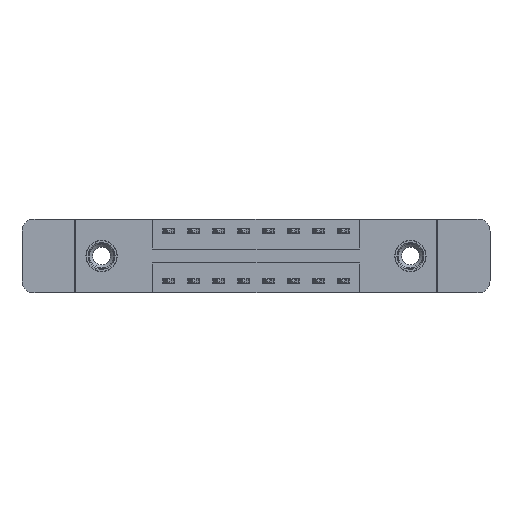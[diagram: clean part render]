
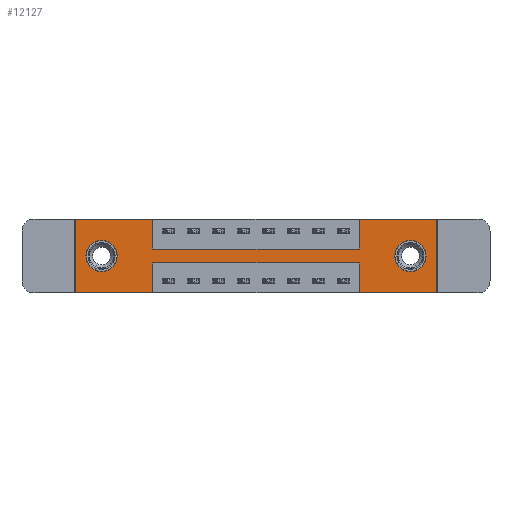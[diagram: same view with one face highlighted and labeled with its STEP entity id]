
A CAD part, front view. The second image highlights one B-rep face of the part: STEP entity #12127.
In plain terms, the highlighted planar face has unit normal (0, -1, 0).
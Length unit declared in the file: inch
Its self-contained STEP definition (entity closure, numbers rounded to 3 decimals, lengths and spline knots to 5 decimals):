
#292 = DIRECTION ( 'NONE',  ( 1., 0., 0. ) ) ;
#681 = CARTESIAN_POINT ( 'NONE',  ( 1.4225, 0., -0.37 ) ) ;
#776 = VERTEX_POINT ( 'NONE', #7445 ) ;
#814 = ORIENTED_EDGE ( 'NONE', *, *, #9265, .T. ) ;
#912 = VECTOR ( 'NONE', #6201, 39.37008 ) ;
#987 = DIRECTION ( 'NONE',  ( 0., 0., -1. ) ) ;
#1143 = PLANE ( 'NONE',  #5718 ) ;
#1169 = CARTESIAN_POINT ( 'NONE',  ( 0., 0., 0. ) ) ;
#1206 = DIRECTION ( 'NONE',  ( -1., 0., 0. ) ) ;
#1479 = EDGE_CURVE ( 'NONE', #11571, #13150, #12919, .T. ) ;
#1709 = ORIENTED_EDGE ( 'NONE', *, *, #5770, .F. ) ;
#1816 = DIRECTION ( 'NONE',  ( 0., 1., 0. ) ) ;
#1830 = ORIENTED_EDGE ( 'NONE', *, *, #4069, .F. ) ;
#1950 = VERTEX_POINT ( 'NONE', #3551 ) ;
#2066 = EDGE_CURVE ( 'NONE', #13150, #11571, #7248, .T. ) ;
#2183 = DIRECTION ( 'NONE',  ( 0., 0., -1. ) ) ;
#2210 = ORIENTED_EDGE ( 'NONE', *, *, #11761, .F. ) ;
#2298 = AXIS2_PLACEMENT_3D ( 'NONE', #3751, #12942, #4683 ) ;
#2528 = CARTESIAN_POINT ( 'NONE',  ( 0., 0., -0.37 ) ) ;
#2551 = DIRECTION ( 'NONE',  ( 0., -1., 0. ) ) ;
#3157 = EDGE_CURVE ( 'NONE', #13590, #13676, #3635, .T. ) ;
#3360 = CARTESIAN_POINT ( 'NONE',  ( 0.1325, 0., -0.107 ) ) ;
#3379 = VERTEX_POINT ( 'NONE', #6526 ) ;
#3422 = CIRCLE ( 'NONE', #5685, 0.078 ) ;
#3471 = VECTOR ( 'NONE', #6344, 39.37008 ) ;
#3551 = CARTESIAN_POINT ( 'NONE',  ( 0.3875, 0., -0.37 ) ) ;
#3635 = LINE ( 'NONE', #8270, #8037 ) ;
#3661 = VECTOR ( 'NONE', #12760, 39.37008 ) ;
#3684 = LINE ( 'NONE', #7225, #14088 ) ;
#3749 = AXIS2_PLACEMENT_3D ( 'NONE', #9615, #14564, #7372 ) ;
#3751 = CARTESIAN_POINT ( 'NONE',  ( 0.1325, 0., -0.185 ) ) ;
#4069 = EDGE_CURVE ( 'NONE', #776, #15091, #3684, .T. ) ;
#4244 = DIRECTION ( 'NONE',  ( 0., 0., 1. ) ) ;
#4287 = EDGE_CURVE ( 'NONE', #8488, #13590, #7455, .T. ) ;
#4439 = ORIENTED_EDGE ( 'NONE', *, *, #14115, .F. ) ;
#4582 = CARTESIAN_POINT ( 'NONE',  ( 1.4225, 0., 0. ) ) ;
#4631 = CARTESIAN_POINT ( 'NONE',  ( 1.4225, 0., 0. ) ) ;
#4674 = LINE ( 'NONE', #10520, #13749 ) ;
#4681 = VECTOR ( 'NONE', #292, 39.37008 ) ;
#4683 = DIRECTION ( 'NONE',  ( 0., 0., 1. ) ) ;
#4753 = CARTESIAN_POINT ( 'NONE',  ( 0., 0., -0.37 ) ) ;
#4797 = VERTEX_POINT ( 'NONE', #4631 ) ;
#4828 = ORIENTED_EDGE ( 'NONE', *, *, #12594, .F. ) ;
#4850 = LINE ( 'NONE', #8381, #8922 ) ;
#5213 = VERTEX_POINT ( 'NONE', #3360 ) ;
#5369 = VERTEX_POINT ( 'NONE', #9388 ) ;
#5603 = EDGE_CURVE ( 'NONE', #1950, #11584, #5709, .T. ) ;
#5670 = VERTEX_POINT ( 'NONE', #13775 ) ;
#5685 = AXIS2_PLACEMENT_3D ( 'NONE', #15165, #1816, #4244 ) ;
#5709 = LINE ( 'NONE', #14878, #10651 ) ;
#5718 = AXIS2_PLACEMENT_3D ( 'NONE', #4753, #2551, #10680 ) ;
#5770 = EDGE_CURVE ( 'NONE', #5670, #3379, #4674, .T. ) ;
#5925 = ORIENTED_EDGE ( 'NONE', *, *, #7505, .T. ) ;
#6201 = DIRECTION ( 'NONE',  ( 0., 0., 1. ) ) ;
#6270 = EDGE_CURVE ( 'NONE', #9476, #4797, #15256, .T. ) ;
#6344 = DIRECTION ( 'NONE',  ( 0., 0., 1. ) ) ;
#6373 = DIRECTION ( 'NONE',  ( 0., 1., 0. ) ) ;
#6526 = CARTESIAN_POINT ( 'NONE',  ( 1.81, 0., -0.37 ) ) ;
#6554 = EDGE_LOOP ( 'NONE', ( #11236, #10657 ) ) ;
#7031 = DIRECTION ( 'NONE',  ( 0., 0., 1. ) ) ;
#7146 = LINE ( 'NONE', #1169, #3471 ) ;
#7225 = CARTESIAN_POINT ( 'NONE',  ( 0.3875, 0., 0. ) ) ;
#7248 = CIRCLE ( 'NONE', #14914, 0.078 ) ;
#7279 = ORIENTED_EDGE ( 'NONE', *, *, #14817, .F. ) ;
#7372 = DIRECTION ( 'NONE',  ( 0., 0., -1. ) ) ;
#7409 = CARTESIAN_POINT ( 'NONE',  ( 1.6775, 0., -0.185 ) ) ;
#7445 = CARTESIAN_POINT ( 'NONE',  ( 0.3875, 0., 0. ) ) ;
#7455 = LINE ( 'NONE', #13542, #912 ) ;
#7505 = EDGE_CURVE ( 'NONE', #5213, #5369, #9033, .T. ) ;
#7534 = CARTESIAN_POINT ( 'NONE',  ( 1.4225, 0., -0.15 ) ) ;
#7692 = ORIENTED_EDGE ( 'NONE', *, *, #5603, .F. ) ;
#8037 = VECTOR ( 'NONE', #9661, 39.37008 ) ;
#8116 = LINE ( 'NONE', #12607, #3661 ) ;
#8212 = CARTESIAN_POINT ( 'NONE',  ( 1.6775, 0., -0.263 ) ) ;
#8226 = DIRECTION ( 'NONE',  ( 0., 0., -1. ) ) ;
#8270 = CARTESIAN_POINT ( 'NONE',  ( 0.3875, 0., -0.22 ) ) ;
#8381 = CARTESIAN_POINT ( 'NONE',  ( 0.3875, 0., -0.37 ) ) ;
#8488 = VERTEX_POINT ( 'NONE', #681 ) ;
#8575 = LINE ( 'NONE', #2528, #8892 ) ;
#8584 = VECTOR ( 'NONE', #7031, 39.37008 ) ;
#8851 = DIRECTION ( 'NONE',  ( 0., 0., -1. ) ) ;
#8892 = VECTOR ( 'NONE', #1206, 39.37008 ) ;
#8922 = VECTOR ( 'NONE', #8226, 39.37008 ) ;
#8927 = EDGE_CURVE ( 'NONE', #4797, #5670, #8116, .T. ) ;
#9033 = CIRCLE ( 'NONE', #2298, 0.078 ) ;
#9265 = EDGE_CURVE ( 'NONE', #5369, #5213, #3422, .T. ) ;
#9388 = CARTESIAN_POINT ( 'NONE',  ( 0.1325, 0., -0.263 ) ) ;
#9476 = VERTEX_POINT ( 'NONE', #7534 ) ;
#9492 = EDGE_LOOP ( 'NONE', ( #5925, #814 ) ) ;
#9597 = CARTESIAN_POINT ( 'NONE',  ( 0.3875, 0., -0.22 ) ) ;
#9615 = CARTESIAN_POINT ( 'NONE',  ( 1.6775, 0., -0.185 ) ) ;
#9629 = EDGE_LOOP ( 'NONE', ( #7279, #9812, #11329, #4439, #1709, #13798, #12072, #4828, #1830, #13626, #2210, #7692 ) ) ;
#9661 = DIRECTION ( 'NONE',  ( -1., 0., 0. ) ) ;
#9812 = ORIENTED_EDGE ( 'NONE', *, *, #3157, .F. ) ;
#10175 = LINE ( 'NONE', #11498, #11233 ) ;
#10444 = CARTESIAN_POINT ( 'NONE',  ( 0., 0., 0. ) ) ;
#10520 = CARTESIAN_POINT ( 'NONE',  ( 1.81, 0., 0. ) ) ;
#10651 = VECTOR ( 'NONE', #15112, 39.37008 ) ;
#10657 = ORIENTED_EDGE ( 'NONE', *, *, #2066, .T. ) ;
#10680 = DIRECTION ( 'NONE',  ( 0., 0., -1. ) ) ;
#11003 = CARTESIAN_POINT ( 'NONE',  ( 0., 0., 0. ) ) ;
#11025 = CARTESIAN_POINT ( 'NONE',  ( 0., 0., -0.37 ) ) ;
#11233 = VECTOR ( 'NONE', #15068, 39.37008 ) ;
#11236 = ORIENTED_EDGE ( 'NONE', *, *, #1479, .T. ) ;
#11329 = ORIENTED_EDGE ( 'NONE', *, *, #4287, .F. ) ;
#11454 = CARTESIAN_POINT ( 'NONE',  ( 0.3875, 0., -0.15 ) ) ;
#11498 = CARTESIAN_POINT ( 'NONE',  ( 0.3875, 0., -0.15 ) ) ;
#11571 = VERTEX_POINT ( 'NONE', #14743 ) ;
#11584 = VERTEX_POINT ( 'NONE', #11025 ) ;
#11708 = CARTESIAN_POINT ( 'NONE',  ( 1.4225, 0., -0.22 ) ) ;
#11761 = EDGE_CURVE ( 'NONE', #11584, #13017, #7146, .T. ) ;
#12072 = ORIENTED_EDGE ( 'NONE', *, *, #6270, .F. ) ;
#12127 = ADVANCED_FACE ( 'NONE', ( #13010, #14419, #13243 ), #1143, .T. ) ;
#12594 = EDGE_CURVE ( 'NONE', #15091, #9476, #10175, .T. ) ;
#12607 = CARTESIAN_POINT ( 'NONE',  ( 0., 0., 0. ) ) ;
#12760 = DIRECTION ( 'NONE',  ( 1., 0., 0. ) ) ;
#12919 = CIRCLE ( 'NONE', #3749, 0.078 ) ;
#12942 = DIRECTION ( 'NONE',  ( 0., 1., 0. ) ) ;
#13010 = FACE_BOUND ( 'NONE', #6554, .T. ) ;
#13017 = VERTEX_POINT ( 'NONE', #10444 ) ;
#13150 = VERTEX_POINT ( 'NONE', #8212 ) ;
#13243 = FACE_OUTER_BOUND ( 'NONE', #9629, .T. ) ;
#13542 = CARTESIAN_POINT ( 'NONE',  ( 1.4225, 0., -0.37 ) ) ;
#13590 = VERTEX_POINT ( 'NONE', #11708 ) ;
#13626 = ORIENTED_EDGE ( 'NONE', *, *, #14933, .F. ) ;
#13676 = VERTEX_POINT ( 'NONE', #9597 ) ;
#13749 = VECTOR ( 'NONE', #987, 39.37008 ) ;
#13775 = CARTESIAN_POINT ( 'NONE',  ( 1.81, 0., 0. ) ) ;
#13798 = ORIENTED_EDGE ( 'NONE', *, *, #8927, .F. ) ;
#14088 = VECTOR ( 'NONE', #2183, 39.37008 ) ;
#14115 = EDGE_CURVE ( 'NONE', #3379, #8488, #8575, .T. ) ;
#14419 = FACE_BOUND ( 'NONE', #9492, .T. ) ;
#14433 = LINE ( 'NONE', #11003, #4681 ) ;
#14564 = DIRECTION ( 'NONE',  ( 0., 1., 0. ) ) ;
#14743 = CARTESIAN_POINT ( 'NONE',  ( 1.6775, 0., -0.107 ) ) ;
#14817 = EDGE_CURVE ( 'NONE', #13676, #1950, #4850, .T. ) ;
#14878 = CARTESIAN_POINT ( 'NONE',  ( 0., 0., -0.37 ) ) ;
#14914 = AXIS2_PLACEMENT_3D ( 'NONE', #7409, #6373, #8851 ) ;
#14933 = EDGE_CURVE ( 'NONE', #13017, #776, #14433, .T. ) ;
#15068 = DIRECTION ( 'NONE',  ( 1., 0., 0. ) ) ;
#15091 = VERTEX_POINT ( 'NONE', #11454 ) ;
#15112 = DIRECTION ( 'NONE',  ( -1., 0., 0. ) ) ;
#15165 = CARTESIAN_POINT ( 'NONE',  ( 0.1325, 0., -0.185 ) ) ;
#15256 = LINE ( 'NONE', #4582, #8584 ) ;
